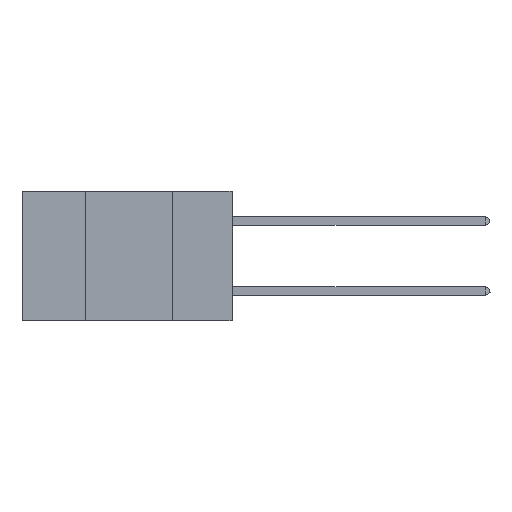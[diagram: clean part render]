
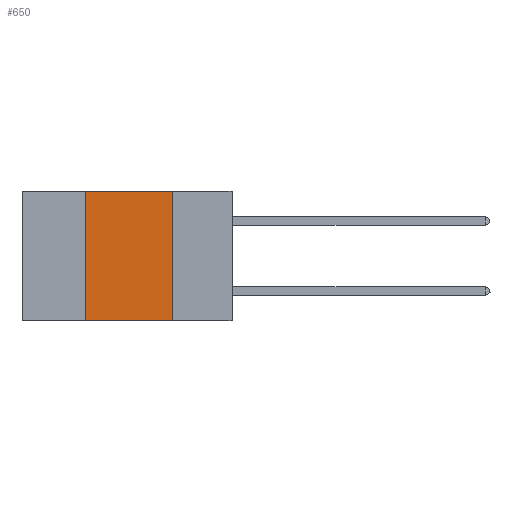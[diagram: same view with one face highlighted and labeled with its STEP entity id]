
A CAD part, left-side view. The second image highlights one B-rep face of the part: STEP entity #650.
In plain terms, the highlighted planar face has unit normal (-1, 0, 0).
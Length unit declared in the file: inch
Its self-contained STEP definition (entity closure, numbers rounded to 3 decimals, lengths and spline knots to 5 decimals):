
#96 = CARTESIAN_POINT ( 'NONE',  ( 0., 0.42, 0. ) ) ;
#581 = VECTOR ( 'NONE', #2550, 39.37008 ) ;
#650 = ADVANCED_FACE ( 'NONE', ( #1295 ), #985, .F. ) ;
#709 = CARTESIAN_POINT ( 'NONE',  ( 0., 0.6, 0. ) ) ;
#985 = PLANE ( 'NONE',  #10986 ) ;
#1295 = FACE_OUTER_BOUND ( 'NONE', #8539, .T. ) ;
#1385 = ORIENTED_EDGE ( 'NONE', *, *, #9483, .F. ) ;
#1607 = CARTESIAN_POINT ( 'NONE',  ( 0., 0.6, -0.37 ) ) ;
#1712 = LINE ( 'NONE', #709, #10752 ) ;
#2015 = DIRECTION ( 'NONE',  ( 0., 0., 1. ) ) ;
#2208 = ORIENTED_EDGE ( 'NONE', *, *, #10038, .T. ) ;
#2550 = DIRECTION ( 'NONE',  ( 0., -1., 0. ) ) ;
#2695 = VECTOR ( 'NONE', #7623, 39.37008 ) ;
#2879 = LINE ( 'NONE', #1607, #581 ) ;
#3052 = DIRECTION ( 'NONE',  ( 1., 0., 0. ) ) ;
#3865 = CARTESIAN_POINT ( 'NONE',  ( 0., 0.6, 0. ) ) ;
#4514 = VERTEX_POINT ( 'NONE', #8298 ) ;
#4900 = VERTEX_POINT ( 'NONE', #6531 ) ;
#5837 = CARTESIAN_POINT ( 'NONE',  ( 0., 0.42, -0.37 ) ) ;
#5933 = DIRECTION ( 'NONE',  ( 0., 0., -1. ) ) ;
#6314 = EDGE_CURVE ( 'NONE', #7882, #4900, #1712, .T. ) ;
#6531 = CARTESIAN_POINT ( 'NONE',  ( 0., 0.17, 0. ) ) ;
#6608 = VECTOR ( 'NONE', #2015, 39.37008 ) ;
#6629 = CARTESIAN_POINT ( 'NONE',  ( 0., 0.17, 0. ) ) ;
#7138 = LINE ( 'NONE', #6629, #2695 ) ;
#7303 = EDGE_CURVE ( 'NONE', #11304, #7882, #11805, .T. ) ;
#7623 = DIRECTION ( 'NONE',  ( 0., 0., -1. ) ) ;
#7882 = VERTEX_POINT ( 'NONE', #10990 ) ;
#8184 = ORIENTED_EDGE ( 'NONE', *, *, #6314, .F. ) ;
#8298 = CARTESIAN_POINT ( 'NONE',  ( 0., 0.17, -0.37 ) ) ;
#8539 = EDGE_LOOP ( 'NONE', ( #1385, #8184, #9054, #2208 ) ) ;
#9054 = ORIENTED_EDGE ( 'NONE', *, *, #7303, .F. ) ;
#9483 = EDGE_CURVE ( 'NONE', #4900, #4514, #7138, .T. ) ;
#10038 = EDGE_CURVE ( 'NONE', #11304, #4514, #2879, .T. ) ;
#10752 = VECTOR ( 'NONE', #11571, 39.37008 ) ;
#10986 = AXIS2_PLACEMENT_3D ( 'NONE', #3865, #3052, #5933 ) ;
#10990 = CARTESIAN_POINT ( 'NONE',  ( 0., 0.42, 0. ) ) ;
#11304 = VERTEX_POINT ( 'NONE', #5837 ) ;
#11571 = DIRECTION ( 'NONE',  ( 0., -1., 0. ) ) ;
#11805 = LINE ( 'NONE', #96, #6608 ) ;
